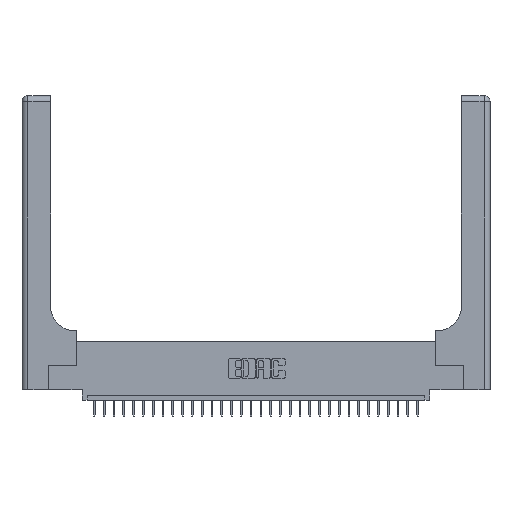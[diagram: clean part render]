
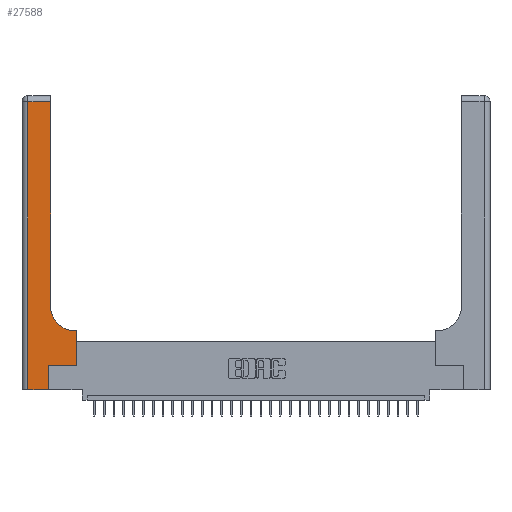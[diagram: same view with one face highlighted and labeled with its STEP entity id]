
A CAD part, top view. The second image highlights one B-rep face of the part: STEP entity #27588.
In plain terms, the highlighted planar face has unit normal (0, 0, 1).
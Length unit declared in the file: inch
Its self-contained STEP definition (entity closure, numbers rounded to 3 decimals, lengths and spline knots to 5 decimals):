
#605 = ORIENTED_EDGE ( 'NONE', *, *, #15375, .T. ) ;
#882 = DIRECTION ( 'NONE',  ( -1., 0., 0. ) ) ;
#1061 = VECTOR ( 'NONE', #14926, 39.37008 ) ;
#1711 = EDGE_CURVE ( 'NONE', #5154, #23708, #12042, .T. ) ;
#1838 = DIRECTION ( 'NONE',  ( 0., 0., -1. ) ) ;
#2104 = LINE ( 'NONE', #4902, #15237 ) ;
#2203 = EDGE_LOOP ( 'NONE', ( #19390, #5753, #605, #14958, #12539, #30208, #10936, #29747, #30605 ) ) ;
#2574 = EDGE_CURVE ( 'NONE', #26210, #25600, #25809, .T. ) ;
#3676 = DIRECTION ( 'NONE',  ( -1., 0., 0. ) ) ;
#4057 = VECTOR ( 'NONE', #20402, 39.37008 ) ;
#4146 = VECTOR ( 'NONE', #13292, 39.37008 ) ;
#4329 = DIRECTION ( 'NONE',  ( 1., 0., 0. ) ) ;
#4902 = CARTESIAN_POINT ( 'NONE',  ( 0.269, 0., 0.37 ) ) ;
#5013 = CARTESIAN_POINT ( 'NONE',  ( 0.06, 2.94, 0.37 ) ) ;
#5154 = VERTEX_POINT ( 'NONE', #19274 ) ;
#5753 = ORIENTED_EDGE ( 'NONE', *, *, #22975, .T. ) ;
#7081 = CARTESIAN_POINT ( 'NONE',  ( 0.5415, 0.6, 0.37 ) ) ;
#7518 = EDGE_CURVE ( 'NONE', #17753, #22852, #24508, .T. ) ;
#8434 = DIRECTION ( 'NONE',  ( 0., 0., -1. ) ) ;
#8801 = CARTESIAN_POINT ( 'NONE',  ( 0.5585, 0.25, 0.37 ) ) ;
#10464 = CARTESIAN_POINT ( 'NONE',  ( 0.2915, 2.94, 0.37 ) ) ;
#10755 = FACE_OUTER_BOUND ( 'NONE', #2203, .T. ) ;
#10936 = ORIENTED_EDGE ( 'NONE', *, *, #16452, .T. ) ;
#11489 = LINE ( 'NONE', #25669, #4146 ) ;
#12042 = LINE ( 'NONE', #30672, #13934 ) ;
#12539 = ORIENTED_EDGE ( 'NONE', *, *, #22725, .T. ) ;
#13089 = CARTESIAN_POINT ( 'NONE',  ( 0., 2.94, 0.37 ) ) ;
#13292 = DIRECTION ( 'NONE',  ( 0., 1., 0. ) ) ;
#13428 = EDGE_CURVE ( 'NONE', #23708, #29787, #22983, .T. ) ;
#13534 = VERTEX_POINT ( 'NONE', #5013 ) ;
#13934 = VECTOR ( 'NONE', #25766, 39.37008 ) ;
#14238 = VERTEX_POINT ( 'NONE', #10464 ) ;
#14675 = CARTESIAN_POINT ( 'NONE',  ( 0.269, 0.25, 0.37 ) ) ;
#14926 = DIRECTION ( 'NONE',  ( 0., -1., 0. ) ) ;
#14958 = ORIENTED_EDGE ( 'NONE', *, *, #7518, .T. ) ;
#15237 = VECTOR ( 'NONE', #22233, 39.37008 ) ;
#15375 = EDGE_CURVE ( 'NONE', #13534, #17753, #26171, .T. ) ;
#15597 = VECTOR ( 'NONE', #3676, 39.37008 ) ;
#15677 = CARTESIAN_POINT ( 'NONE',  ( 0., 0., 0.37 ) ) ;
#15731 = EDGE_CURVE ( 'NONE', #29787, #14238, #11489, .T. ) ;
#16452 = EDGE_CURVE ( 'NONE', #25600, #5154, #16474, .T. ) ;
#16474 = LINE ( 'NONE', #8801, #31558 ) ;
#16619 = CARTESIAN_POINT ( 'NONE',  ( 0.5415, 0.85, 0.37 ) ) ;
#17600 = CARTESIAN_POINT ( 'NONE',  ( 0.269, 0., 0.37 ) ) ;
#17753 = VERTEX_POINT ( 'NONE', #24230 ) ;
#19274 = CARTESIAN_POINT ( 'NONE',  ( 0.5585, 0.6, 0.37 ) ) ;
#19336 = CARTESIAN_POINT ( 'NONE',  ( 0.06, 3., 0.37 ) ) ;
#19390 = ORIENTED_EDGE ( 'NONE', *, *, #15731, .T. ) ;
#20402 = DIRECTION ( 'NONE',  ( 1., 0., 0. ) ) ;
#20919 = CARTESIAN_POINT ( 'NONE',  ( 0., 3., 0.37 ) ) ;
#21012 = AXIS2_PLACEMENT_3D ( 'NONE', #16619, #1838, #4329 ) ;
#22233 = DIRECTION ( 'NONE',  ( 0., 1., 0. ) ) ;
#22725 = EDGE_CURVE ( 'NONE', #22852, #26210, #2104, .T. ) ;
#22852 = VERTEX_POINT ( 'NONE', #17600 ) ;
#22975 = EDGE_CURVE ( 'NONE', #14238, #13534, #30666, .T. ) ;
#22983 = CIRCLE ( 'NONE', #21012, 0.25 ) ;
#23219 = PLANE ( 'NONE',  #28822 ) ;
#23708 = VERTEX_POINT ( 'NONE', #7081 ) ;
#24230 = CARTESIAN_POINT ( 'NONE',  ( 0.06, 0., 0.37 ) ) ;
#24508 = LINE ( 'NONE', #15677, #4057 ) ;
#25541 = CARTESIAN_POINT ( 'NONE',  ( 0.269, 0.25, 0.37 ) ) ;
#25600 = VERTEX_POINT ( 'NONE', #28854 ) ;
#25669 = CARTESIAN_POINT ( 'NONE',  ( 0.2915, 3., 0.37 ) ) ;
#25766 = DIRECTION ( 'NONE',  ( -1., 0., 0. ) ) ;
#25809 = LINE ( 'NONE', #25541, #29712 ) ;
#26040 = CARTESIAN_POINT ( 'NONE',  ( 0.2915, 0.85, 0.37 ) ) ;
#26171 = LINE ( 'NONE', #19336, #1061 ) ;
#26210 = VERTEX_POINT ( 'NONE', #14675 ) ;
#27588 = ADVANCED_FACE ( 'NONE', ( #10755 ), #23219, .F. ) ;
#28676 = DIRECTION ( 'NONE',  ( 0., 1., 0. ) ) ;
#28822 = AXIS2_PLACEMENT_3D ( 'NONE', #20919, #8434, #882 ) ;
#28854 = CARTESIAN_POINT ( 'NONE',  ( 0.5585, 0.25, 0.37 ) ) ;
#29712 = VECTOR ( 'NONE', #30544, 39.37008 ) ;
#29747 = ORIENTED_EDGE ( 'NONE', *, *, #1711, .T. ) ;
#29787 = VERTEX_POINT ( 'NONE', #26040 ) ;
#30208 = ORIENTED_EDGE ( 'NONE', *, *, #2574, .T. ) ;
#30544 = DIRECTION ( 'NONE',  ( 1., 0., 0. ) ) ;
#30605 = ORIENTED_EDGE ( 'NONE', *, *, #13428, .T. ) ;
#30666 = LINE ( 'NONE', #13089, #15597 ) ;
#30672 = CARTESIAN_POINT ( 'NONE',  ( 0.2915, 0.6, 0.37 ) ) ;
#31558 = VECTOR ( 'NONE', #28676, 39.37008 ) ;
